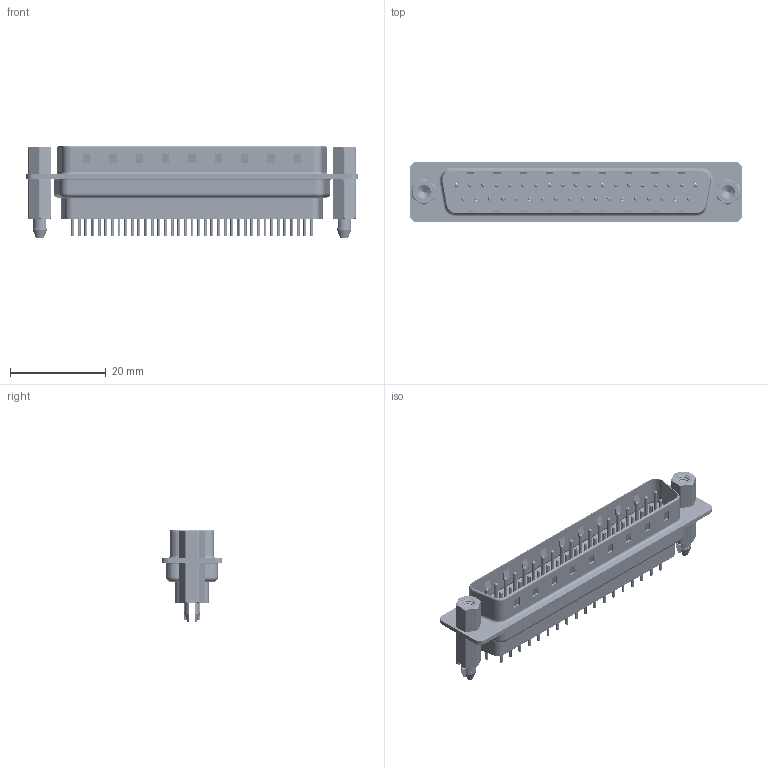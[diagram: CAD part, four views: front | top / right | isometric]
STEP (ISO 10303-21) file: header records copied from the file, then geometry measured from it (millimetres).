
FILE_DESCRIPTION (( 'STEP AP203' ), '1' );
FILE_NAME ('627-037-228-067.STEP', '2020-07-21T17:29:52', ( '' ), ( '' ), 'SwSTEP 2.0', 'SolidWorks 2020', '' );
FILE_SCHEMA (( 'CONFIG_CONTROL_DESIGN' ));
Length unit declared in the file: millimetre
Products named in the file (8): 627 Contact Row 2_28L; 627 Shell Rear_37 Contacts; 627 Shell Front_37 Contacts; 627 Contact Row 1_28L; 627-037-228-067; 627 Housing_37 FF; 627 4-40 Threaded Boardlock_FF; 627 4-40 Hex Standoff
Assembly tree (44 placements, depth 2):
  627-037-228-067
    627 Housing_37 FF
    627 Shell Front_37 Contacts
    627 Shell Rear_37 Contacts
    627 Contact Row 1_28L  x19
    627 Contact Row 2_28L  x18
    627 4-40 Hex Standoff  x2
    627 4-40 Threaded Boardlock_FF  x2
Bounding box: 69.3 x 12.6 x 19.4 mm (x, y, z)
Volume: 4949.7 mm3; surface area: 13243.5 mm2
Topology: 45 solids, 45 shells, 4405 faces, 11635 edges, 7255 vertices
Faces by surface type: cylinder 1727, plane 1151, torus 1055, cone 406, bspline 66
Entity records: 53547 total; most frequent: CARTESIAN_POINT 24716, DIRECTION 5822, ORIENTED_EDGE 5538, EDGE_CURVE 2769, AXIS2_PLACEMENT_3D 2291, VERTEX_POINT 1788, EDGE_LOOP 1363, VECTOR 1240
